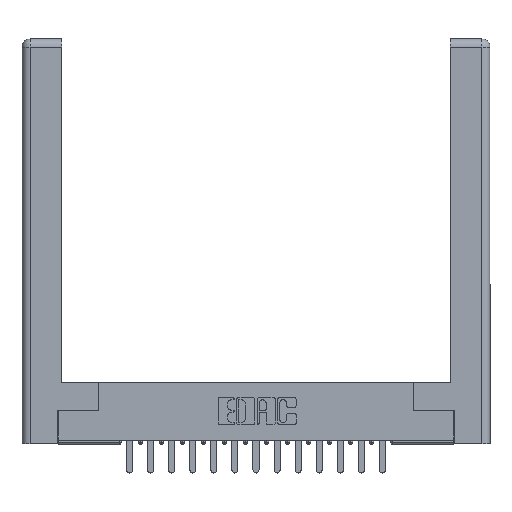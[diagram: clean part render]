
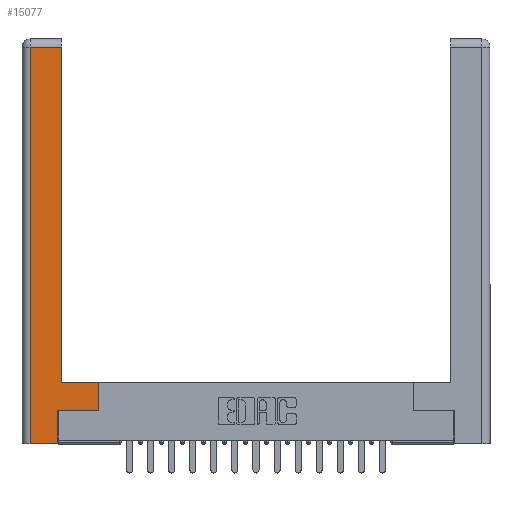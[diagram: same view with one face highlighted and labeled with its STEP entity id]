
A CAD part, top view. The second image highlights one B-rep face of the part: STEP entity #15077.
In plain terms, the highlighted planar face has unit normal (0, 0, 1).
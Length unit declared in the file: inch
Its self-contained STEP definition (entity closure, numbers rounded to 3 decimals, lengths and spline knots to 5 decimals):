
#360 = EDGE_CURVE ( 'NONE', #17096, #3416, #18684, .T. ) ;
#521 = CARTESIAN_POINT ( 'NONE',  ( 0.265, 0., 0. ) ) ;
#648 = VECTOR ( 'NONE', #6761, 39.37008 ) ;
#1025 = CARTESIAN_POINT ( 'NONE',  ( 0.265, 0.245, 0. ) ) ;
#1351 = LINE ( 'NONE', #521, #3289 ) ;
#1420 = EDGE_CURVE ( 'NONE', #4734, #2739, #17205, .T. ) ;
#2739 = VERTEX_POINT ( 'NONE', #12601 ) ;
#2960 = VECTOR ( 'NONE', #19688, 39.37008 ) ;
#3174 = VERTEX_POINT ( 'NONE', #19371 ) ;
#3289 = VECTOR ( 'NONE', #17670, 39.37008 ) ;
#3348 = DIRECTION ( 'NONE',  ( 0., -1., 0. ) ) ;
#3416 = VERTEX_POINT ( 'NONE', #4879 ) ;
#3424 = CARTESIAN_POINT ( 'NONE',  ( 0.0615, 0., 0. ) ) ;
#3489 = VERTEX_POINT ( 'NONE', #6362 ) ;
#3638 = EDGE_CURVE ( 'NONE', #3174, #3489, #1351, .T. ) ;
#4083 = PLANE ( 'NONE',  #14577 ) ;
#4295 = DIRECTION ( 'NONE',  ( -1., 0., 0. ) ) ;
#4384 = EDGE_CURVE ( 'NONE', #2739, #17096, #6908, .T. ) ;
#4628 = EDGE_CURVE ( 'NONE', #3416, #3174, #9862, .T. ) ;
#4734 = VERTEX_POINT ( 'NONE', #9454 ) ;
#4791 = VECTOR ( 'NONE', #8061, 39.37008 ) ;
#4879 = CARTESIAN_POINT ( 'NONE',  ( 0.0615, 2.94, 0. ) ) ;
#4999 = CARTESIAN_POINT ( 'NONE',  ( 0.295, 3., 0. ) ) ;
#5128 = VERTEX_POINT ( 'NONE', #1025 ) ;
#5505 = CARTESIAN_POINT ( 'NONE',  ( 0., 0., 0. ) ) ;
#5791 = VECTOR ( 'NONE', #4295, 39.37008 ) ;
#6108 = ORIENTED_EDGE ( 'NONE', *, *, #4628, .T. ) ;
#6362 = CARTESIAN_POINT ( 'NONE',  ( 0.265, 0., 0. ) ) ;
#6487 = CARTESIAN_POINT ( 'NONE',  ( 0.565, 0.245, 0. ) ) ;
#6492 = LINE ( 'NONE', #19420, #9920 ) ;
#6761 = DIRECTION ( 'NONE',  ( -1., 0., 0. ) ) ;
#6848 = ORIENTED_EDGE ( 'NONE', *, *, #4384, .T. ) ;
#6908 = LINE ( 'NONE', #4999, #17158 ) ;
#8057 = ORIENTED_EDGE ( 'NONE', *, *, #3638, .T. ) ;
#8061 = DIRECTION ( 'NONE',  ( 1., 0., 0. ) ) ;
#8641 = DIRECTION ( 'NONE',  ( -1., 0., 0. ) ) ;
#9454 = CARTESIAN_POINT ( 'NONE',  ( 0.565, 0.45, 0. ) ) ;
#9480 = EDGE_CURVE ( 'NONE', #13387, #4734, #6492, .T. ) ;
#9756 = ORIENTED_EDGE ( 'NONE', *, *, #9918, .T. ) ;
#9862 = LINE ( 'NONE', #3424, #12805 ) ;
#9918 = EDGE_CURVE ( 'NONE', #5128, #13387, #17447, .T. ) ;
#9920 = VECTOR ( 'NONE', #19621, 39.37008 ) ;
#10611 = EDGE_LOOP ( 'NONE', ( #6848, #15542, #6108, #8057, #13885, #9756, #17518, #14174 ) ) ;
#11066 = DIRECTION ( 'NONE',  ( 0., 1., 0. ) ) ;
#11981 = EDGE_CURVE ( 'NONE', #3489, #5128, #19066, .T. ) ;
#12596 = CARTESIAN_POINT ( 'NONE',  ( 0.295, 0.45, 0. ) ) ;
#12601 = CARTESIAN_POINT ( 'NONE',  ( 0.295, 0.45, 0. ) ) ;
#12805 = VECTOR ( 'NONE', #3348, 39.37008 ) ;
#13387 = VERTEX_POINT ( 'NONE', #15156 ) ;
#13615 = CARTESIAN_POINT ( 'NONE',  ( 0.265, 0.245, 0. ) ) ;
#13885 = ORIENTED_EDGE ( 'NONE', *, *, #11981, .T. ) ;
#14174 = ORIENTED_EDGE ( 'NONE', *, *, #1420, .T. ) ;
#14577 = AXIS2_PLACEMENT_3D ( 'NONE', #5505, #14903, #8641 ) ;
#14903 = DIRECTION ( 'NONE',  ( 0., 0., -1. ) ) ;
#15077 = ADVANCED_FACE ( 'NONE', ( #19834 ), #4083, .F. ) ;
#15156 = CARTESIAN_POINT ( 'NONE',  ( 0.565, 0.245, 0. ) ) ;
#15197 = CARTESIAN_POINT ( 'NONE',  ( 0.0615, 2.94, 0. ) ) ;
#15542 = ORIENTED_EDGE ( 'NONE', *, *, #360, .T. ) ;
#15653 = CARTESIAN_POINT ( 'NONE',  ( 0.295, 2.94, 0. ) ) ;
#17096 = VERTEX_POINT ( 'NONE', #15653 ) ;
#17158 = VECTOR ( 'NONE', #11066, 39.37008 ) ;
#17205 = LINE ( 'NONE', #12596, #648 ) ;
#17447 = LINE ( 'NONE', #6487, #4791 ) ;
#17518 = ORIENTED_EDGE ( 'NONE', *, *, #9480, .T. ) ;
#17670 = DIRECTION ( 'NONE',  ( 1., 0., 0. ) ) ;
#18684 = LINE ( 'NONE', #15197, #5791 ) ;
#19066 = LINE ( 'NONE', #13615, #2960 ) ;
#19371 = CARTESIAN_POINT ( 'NONE',  ( 0.0615, 0., 0. ) ) ;
#19420 = CARTESIAN_POINT ( 'NONE',  ( 0.565, 0.45, 0. ) ) ;
#19621 = DIRECTION ( 'NONE',  ( 0., 1., 0. ) ) ;
#19688 = DIRECTION ( 'NONE',  ( 0., 1., 0. ) ) ;
#19834 = FACE_OUTER_BOUND ( 'NONE', #10611, .T. ) ;
